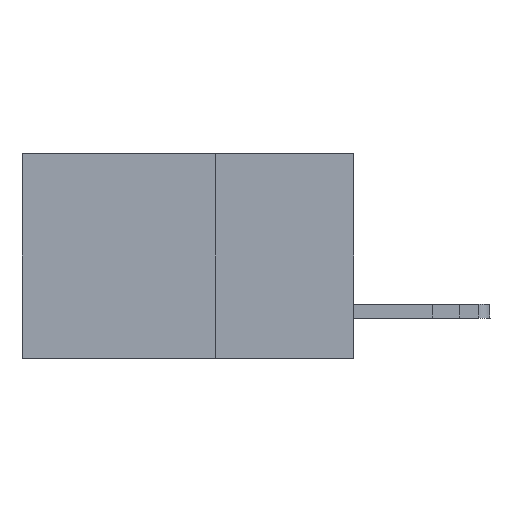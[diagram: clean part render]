
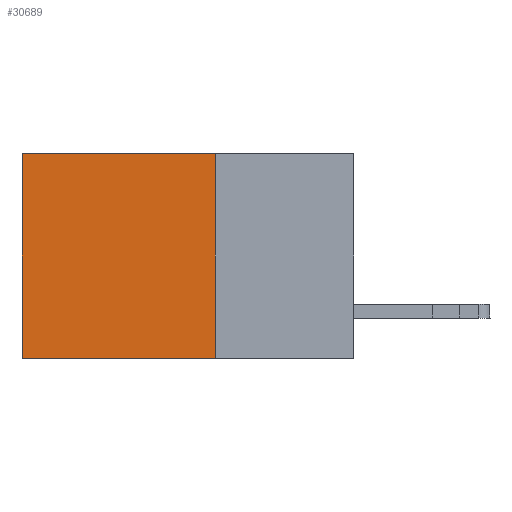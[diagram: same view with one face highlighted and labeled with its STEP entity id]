
A CAD part, left-side view. The second image highlights one B-rep face of the part: STEP entity #30689.
In plain terms, the highlighted planar face has unit normal (-1, 0, 0).
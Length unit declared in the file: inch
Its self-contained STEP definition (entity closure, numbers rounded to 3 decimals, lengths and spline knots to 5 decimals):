
#478 = CARTESIAN_POINT ( 'NONE',  ( 0.2875, 0.25, 0. ) ) ;
#669 = DIRECTION ( 'NONE',  ( 0., 0., -1. ) ) ;
#1351 = LINE ( 'NONE', #15727, #10283 ) ;
#1887 = DIRECTION ( 'NONE',  ( 0., 0., -1. ) ) ;
#1957 = LINE ( 'NONE', #478, #18735 ) ;
#2494 = DIRECTION ( 'NONE',  ( 0., 1., 0. ) ) ;
#2540 = CARTESIAN_POINT ( 'NONE',  ( 0.2875, 0.25, 0. ) ) ;
#3352 = FACE_OUTER_BOUND ( 'NONE', #4657, .T. ) ;
#3784 = LINE ( 'NONE', #9631, #11279 ) ;
#4657 = EDGE_LOOP ( 'NONE', ( #23190, #6442, #15609, #13933 ) ) ;
#5687 = VERTEX_POINT ( 'NONE', #14905 ) ;
#6442 = ORIENTED_EDGE ( 'NONE', *, *, #30073, .F. ) ;
#7588 = EDGE_CURVE ( 'NONE', #8459, #5687, #1351, .T. ) ;
#7889 = DIRECTION ( 'NONE',  ( 1., 0., 0. ) ) ;
#8459 = VERTEX_POINT ( 'NONE', #22623 ) ;
#8849 = VERTEX_POINT ( 'NONE', #13784 ) ;
#9180 = LINE ( 'NONE', #24116, #15061 ) ;
#9631 = CARTESIAN_POINT ( 'NONE',  ( 0.2875, 0.25, -0.37 ) ) ;
#9765 = DIRECTION ( 'NONE',  ( 0., 1., 0. ) ) ;
#10176 = AXIS2_PLACEMENT_3D ( 'NONE', #29306, #7889, #669 ) ;
#10283 = VECTOR ( 'NONE', #1887, 39.37008 ) ;
#11279 = VECTOR ( 'NONE', #2494, 39.37008 ) ;
#13784 = CARTESIAN_POINT ( 'NONE',  ( 0.2875, 0.25, -0.37 ) ) ;
#13933 = ORIENTED_EDGE ( 'NONE', *, *, #19727, .T. ) ;
#13985 = EDGE_CURVE ( 'NONE', #23684, #8849, #1957, .T. ) ;
#14905 = CARTESIAN_POINT ( 'NONE',  ( 0.2875, 0.6, -0.37 ) ) ;
#15061 = VECTOR ( 'NONE', #9765, 39.37008 ) ;
#15609 = ORIENTED_EDGE ( 'NONE', *, *, #13985, .F. ) ;
#15727 = CARTESIAN_POINT ( 'NONE',  ( 0.2875, 0.6, 0. ) ) ;
#18735 = VECTOR ( 'NONE', #29221, 39.37008 ) ;
#19727 = EDGE_CURVE ( 'NONE', #23684, #8459, #9180, .T. ) ;
#22623 = CARTESIAN_POINT ( 'NONE',  ( 0.2875, 0.6, 0. ) ) ;
#23190 = ORIENTED_EDGE ( 'NONE', *, *, #7588, .T. ) ;
#23684 = VERTEX_POINT ( 'NONE', #2540 ) ;
#24116 = CARTESIAN_POINT ( 'NONE',  ( 0.2875, 0.25, 0. ) ) ;
#27095 = PLANE ( 'NONE',  #10176 ) ;
#29221 = DIRECTION ( 'NONE',  ( 0., 0., -1. ) ) ;
#29306 = CARTESIAN_POINT ( 'NONE',  ( 0.2875, 0.25, 0. ) ) ;
#30073 = EDGE_CURVE ( 'NONE', #8849, #5687, #3784, .T. ) ;
#30689 = ADVANCED_FACE ( 'NONE', ( #3352 ), #27095, .F. ) ;
